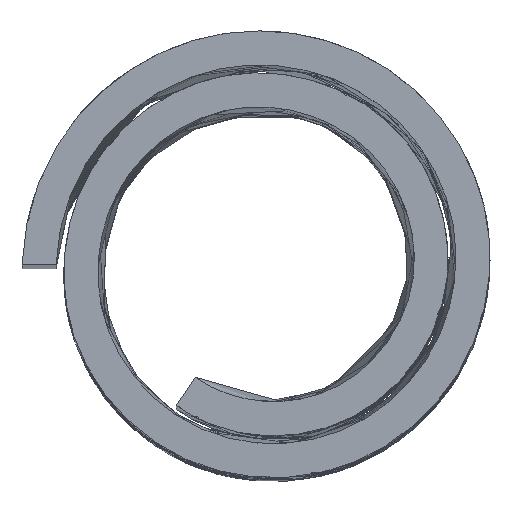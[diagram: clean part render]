
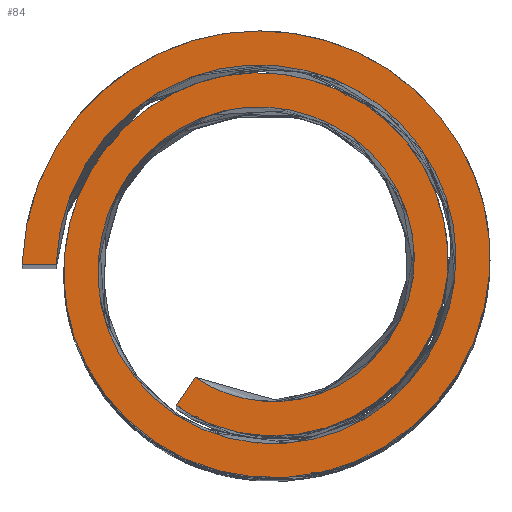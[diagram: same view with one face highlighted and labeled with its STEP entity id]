
A CAD part, top view. The second image highlights one B-rep face of the part: STEP entity #84.
In plain terms, the highlighted planar face has unit normal (0, 0, 1).
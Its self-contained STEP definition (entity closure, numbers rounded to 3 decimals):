
#2 = VECTOR ( 'NONE', #147, 1000. ) ;
#3 = ORIENTED_EDGE ( 'NONE', *, *, #357, .T. ) ;
#18 = VERTEX_POINT ( 'NONE', #363 ) ;
#23 = VERTEX_POINT ( 'NONE', #197 ) ;
#28 = VERTEX_POINT ( 'NONE', #338 ) ;
#39 = VECTOR ( 'NONE', #221, 1000. ) ;
#47 = LINE ( 'NONE', #148, #2 ) ;
#70 = VERTEX_POINT ( 'NONE', #335 ) ;
#72 = ORIENTED_EDGE ( 'NONE', *, *, #369, .F. ) ;
#84 = ADVANCED_FACE ( 'NONE', ( #376 ), #245, .T. ) ;
#119 = CARTESIAN_POINT ( 'NONE',  ( -0.571, -0.892, 7.01 ) ) ;
#120 = CARTESIAN_POINT ( 'NONE',  ( -0.417, -1., 7.01 ) ) ;
#121 = CARTESIAN_POINT ( 'NONE',  ( -0.052, -1.13, 7.01 ) ) ;
#123 = CARTESIAN_POINT ( 'NONE',  ( 0.616, -1.013, 7.01 ) ) ;
#124 = CARTESIAN_POINT ( 'NONE',  ( 1.023, -0.582, 7.01 ) ) ;
#125 = CARTESIAN_POINT ( 'NONE',  ( 1.227, 0.136, 7.01 ) ) ;
#126 = CARTESIAN_POINT ( 'NONE',  ( 0.928, 1.007, 7.01 ) ) ;
#127 = CARTESIAN_POINT ( 'NONE',  ( -0.234, 1.379, 7.01 ) ) ;
#130 = CARTESIAN_POINT ( 'NONE',  ( -1.23, 0.721, 7.01 ) ) ;
#131 = CARTESIAN_POINT ( 'NONE',  ( -1.387, -0.453, 7.01 ) ) ;
#132 = CARTESIAN_POINT ( 'NONE',  ( -0.627, -1.345, 7.01 ) ) ;
#133 = CARTESIAN_POINT ( 'NONE',  ( 0.53, -1.416, 7.01 ) ) ;
#134 = CARTESIAN_POINT ( 'NONE',  ( 1.393, -0.656, 7.01 ) ) ;
#135 = CARTESIAN_POINT ( 'NONE',  ( 1.493, 0.48, 7.01 ) ) ;
#136 = CARTESIAN_POINT ( 'NONE',  ( 0.801, 1.377, 7.01 ) ) ;
#138 = CARTESIAN_POINT ( 'NONE',  ( -0.302, 1.592, 7.01 ) ) ;
#139 = CARTESIAN_POINT ( 'NONE',  ( -1.275, 1.042, 7.01 ) ) ;
#147 = DIRECTION ( 'NONE',  ( -1., 0., 0. ) ) ;
#148 = CARTESIAN_POINT ( 'NONE',  ( -1.333, 0., 7.01 ) ) ;
#172 = CARTESIAN_POINT ( 'NONE',  ( -1.54, 0.35, 7.01 ) ) ;
#193 = CARTESIAN_POINT ( 'NONE',  ( -1.549, 0., 7.01 ) ) ;
#196 = CARTESIAN_POINT ( 'NONE',  ( -0.452, -0.712, 7.01 ) ) ;
#197 = CARTESIAN_POINT ( 'NONE',  ( -0.452, -0.712, 7.01 ) ) ;
#198 = CARTESIAN_POINT ( 'NONE',  ( -0.207, -0.886, 7.01 ) ) ;
#199 = CARTESIAN_POINT ( 'NONE',  ( 0.472, -0.941, 7.01 ) ) ;
#200 = CARTESIAN_POINT ( 'NONE',  ( 1.082, -0.126, 7.01 ) ) ;
#201 = CARTESIAN_POINT ( 'NONE',  ( 0.758, 0.824, 7.01 ) ) ;
#204 = CARTESIAN_POINT ( 'NONE',  ( -0.191, 1.136, 7.01 ) ) ;
#205 = CARTESIAN_POINT ( 'NONE',  ( -1.02, 0.598, 7.01 ) ) ;
#207 = CARTESIAN_POINT ( 'NONE',  ( -1.156, -0.378, 7.01 ) ) ;
#209 = CARTESIAN_POINT ( 'NONE',  ( -0.526, -1.126, 7.01 ) ) ;
#210 = CARTESIAN_POINT ( 'NONE',  ( 0.446, -1.192, 7.01 ) ) ;
#211 = CARTESIAN_POINT ( 'NONE',  ( 1.177, -0.555, 7.01 ) ) ;
#212 = CARTESIAN_POINT ( 'NONE',  ( 1.268, 0.407, 7.01 ) ) ;
#213 = CARTESIAN_POINT ( 'NONE',  ( 0.683, 1.173, 7.01 ) ) ;
#214 = CARTESIAN_POINT ( 'NONE',  ( -0.257, 1.362, 7.01 ) ) ;
#216 = CARTESIAN_POINT ( 'NONE',  ( -1.093, 0.895, 7.01 ) ) ;
#221 = DIRECTION ( 'NONE',  ( 0.552, 0.834, 0. ) ) ;
#222 = CARTESIAN_POINT ( 'NONE',  ( -1.333, 0., 7.01 ) ) ;
#228 = CARTESIAN_POINT ( 'NONE',  ( -0.452, -0.712, 7.01 ) ) ;
#231 = CARTESIAN_POINT ( 'NONE',  ( -1.324, 0.301, 7.01 ) ) ;
#236 = AXIS2_PLACEMENT_3D ( 'NONE', #333, #239, #238 ) ;
#238 = DIRECTION ( 'NONE',  ( 1., 0., 0. ) ) ;
#239 = DIRECTION ( 'NONE',  ( 0., 0., 1. ) ) ;
#242 = EDGE_LOOP ( 'NONE', ( #72, #3, #269, #257 ) ) ;
#245 = PLANE ( 'NONE',  #236 ) ;
#257 = ORIENTED_EDGE ( 'NONE', *, *, #370, .F. ) ;
#261 = B_SPLINE_CURVE_WITH_KNOTS ( 'NONE', 3,
 ( #193, #172, #139, #138, #136, #135, #134, #133, #132, #131, #130, #127, #126, #125, #124, #123, #121, #120, #119 ),
 .UNSPECIFIED., .F., .F.,
 ( 4, 1, 1, 1, 1, 1, 1, 1, 1, 1, 1, 1, 1, 1, 1, 1, 4 ),
 ( 0., 0.09, 0.179, 0.269, 0.358, 0.448, 0.537, 0.627, 0.717, 0.806, 0.896, 0.985, 1.075, 1.097, 1.165, 1.209, 1.254 ),
 .UNSPECIFIED. ) ;
#269 = ORIENTED_EDGE ( 'NONE', *, *, #323, .F. ) ;
#323 = EDGE_CURVE ( 'NONE', #70, #23, #344, .T. ) ;
#333 = CARTESIAN_POINT ( 'NONE',  ( -1.549, 0., 7.01 ) ) ;
#335 = CARTESIAN_POINT ( 'NONE',  ( -0.571, -0.892, 7.01 ) ) ;
#338 = CARTESIAN_POINT ( 'NONE',  ( -1.333, 0., 7.01 ) ) ;
#344 = LINE ( 'NONE', #228, #39 ) ;
#357 = EDGE_CURVE ( 'NONE', #28, #23, #380, .T. ) ;
#363 = CARTESIAN_POINT ( 'NONE',  ( -1.549, 0., 7.01 ) ) ;
#369 = EDGE_CURVE ( 'NONE', #28, #18, #47, .T. ) ;
#370 = EDGE_CURVE ( 'NONE', #18, #70, #261, .T. ) ;
#376 = FACE_OUTER_BOUND ( 'NONE', #242, .T. ) ;
#380 = B_SPLINE_CURVE_WITH_KNOTS ( 'NONE', 3,
 ( #222, #231, #216, #214, #213, #212, #211, #210, #209, #207, #205, #204, #201, #200, #199, #198, #196 ),
 .UNSPECIFIED., .F., .F.,
 ( 4, 1, 1, 1, 1, 1, 1, 1, 1, 1, 1, 1, 1, 1, 4 ),
 ( 0., 0.09, 0.179, 0.269, 0.358, 0.448, 0.537, 0.627, 0.717, 0.806, 0.896, 0.985, 1.075, 1.165, 1.254 ),
 .UNSPECIFIED. ) ;
